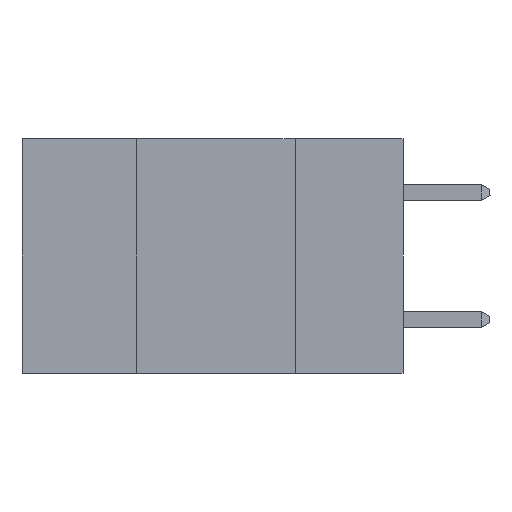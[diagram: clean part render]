
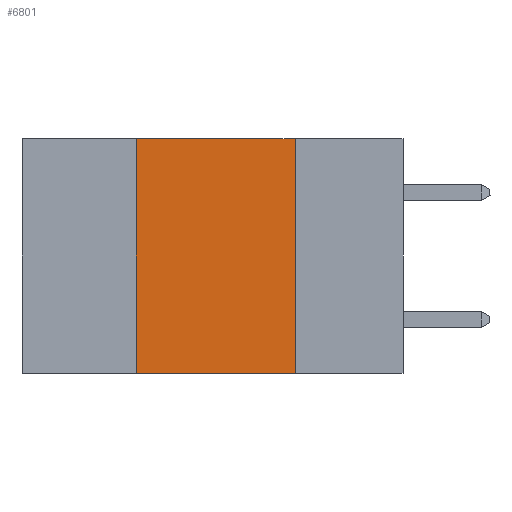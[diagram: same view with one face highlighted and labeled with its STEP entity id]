
A CAD part, left-side view. The second image highlights one B-rep face of the part: STEP entity #6801.
In plain terms, the highlighted planar face has unit normal (-1, 0, 0).
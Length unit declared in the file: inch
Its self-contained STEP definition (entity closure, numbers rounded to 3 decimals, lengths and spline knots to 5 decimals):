
#582 = LINE ( 'NONE', #15882, #4328 ) ;
#913 = VECTOR ( 'NONE', #3639, 39.37008 ) ;
#1147 = CARTESIAN_POINT ( 'NONE',  ( 0., 0.17, -0.37 ) ) ;
#2246 = VECTOR ( 'NONE', #13852, 39.37008 ) ;
#2286 = VECTOR ( 'NONE', #3165, 39.37008 ) ;
#3165 = DIRECTION ( 'NONE',  ( 0., 0., -1. ) ) ;
#3218 = CARTESIAN_POINT ( 'NONE',  ( 0., 0.42, 0. ) ) ;
#3277 = VERTEX_POINT ( 'NONE', #13451 ) ;
#3409 = LINE ( 'NONE', #3218, #2246 ) ;
#3639 = DIRECTION ( 'NONE',  ( 0., -1., 0. ) ) ;
#4328 = VECTOR ( 'NONE', #8359, 39.37008 ) ;
#4622 = CARTESIAN_POINT ( 'NONE',  ( 0., 0.17, 0. ) ) ;
#4828 = EDGE_CURVE ( 'NONE', #3277, #11553, #3409, .T. ) ;
#4994 = ORIENTED_EDGE ( 'NONE', *, *, #8855, .F. ) ;
#5209 = LINE ( 'NONE', #6557, #913 ) ;
#6368 = VERTEX_POINT ( 'NONE', #9941 ) ;
#6557 = CARTESIAN_POINT ( 'NONE',  ( 0., 0.6, 0. ) ) ;
#6801 = ADVANCED_FACE ( 'NONE', ( #18790 ), #13030, .F. ) ;
#7055 = EDGE_LOOP ( 'NONE', ( #16135, #4994, #13805, #9508 ) ) ;
#8359 = DIRECTION ( 'NONE',  ( 0., -1., 0. ) ) ;
#8447 = CARTESIAN_POINT ( 'NONE',  ( 0., 0.6, 0. ) ) ;
#8855 = EDGE_CURVE ( 'NONE', #11553, #6368, #5209, .T. ) ;
#9255 = EDGE_CURVE ( 'NONE', #3277, #18742, #582, .T. ) ;
#9472 = CARTESIAN_POINT ( 'NONE',  ( 0., 0.42, 0. ) ) ;
#9508 = ORIENTED_EDGE ( 'NONE', *, *, #9255, .T. ) ;
#9941 = CARTESIAN_POINT ( 'NONE',  ( 0., 0.17, 0. ) ) ;
#11553 = VERTEX_POINT ( 'NONE', #9472 ) ;
#12947 = DIRECTION ( 'NONE',  ( 1., 0., 0. ) ) ;
#13030 = PLANE ( 'NONE',  #16535 ) ;
#13451 = CARTESIAN_POINT ( 'NONE',  ( 0., 0.42, -0.37 ) ) ;
#13805 = ORIENTED_EDGE ( 'NONE', *, *, #4828, .F. ) ;
#13852 = DIRECTION ( 'NONE',  ( 0., 0., 1. ) ) ;
#13950 = EDGE_CURVE ( 'NONE', #6368, #18742, #14861, .T. ) ;
#14861 = LINE ( 'NONE', #4622, #2286 ) ;
#15882 = CARTESIAN_POINT ( 'NONE',  ( 0., 0.6, -0.37 ) ) ;
#16135 = ORIENTED_EDGE ( 'NONE', *, *, #13950, .F. ) ;
#16535 = AXIS2_PLACEMENT_3D ( 'NONE', #8447, #12947, #18879 ) ;
#18742 = VERTEX_POINT ( 'NONE', #1147 ) ;
#18790 = FACE_OUTER_BOUND ( 'NONE', #7055, .T. ) ;
#18879 = DIRECTION ( 'NONE',  ( 0., 0., -1. ) ) ;
